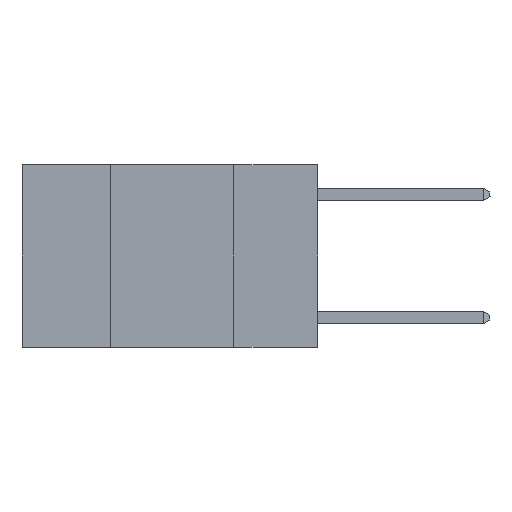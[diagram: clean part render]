
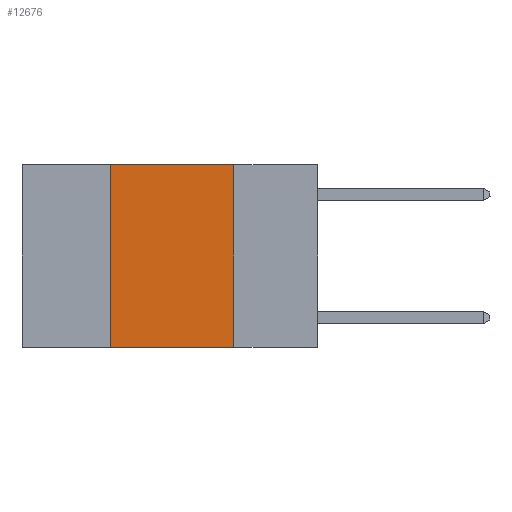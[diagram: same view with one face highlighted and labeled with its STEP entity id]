
A CAD part, left-side view. The second image highlights one B-rep face of the part: STEP entity #12676.
In plain terms, the highlighted planar face has unit normal (-1, 0, 0).
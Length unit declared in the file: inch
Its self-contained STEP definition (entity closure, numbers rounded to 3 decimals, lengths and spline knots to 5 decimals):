
#191 = DIRECTION ( 'NONE',  ( 0., -1., 0. ) ) ;
#1680 = DIRECTION ( 'NONE',  ( 0., 0., 1. ) ) ;
#1792 = ORIENTED_EDGE ( 'NONE', *, *, #13717, .F. ) ;
#2006 = CARTESIAN_POINT ( 'NONE',  ( 0., 0.17, 0. ) ) ;
#2585 = LINE ( 'NONE', #7624, #8014 ) ;
#2943 = FACE_OUTER_BOUND ( 'NONE', #9807, .T. ) ;
#3762 = VECTOR ( 'NONE', #191, 39.37008 ) ;
#3884 = DIRECTION ( 'NONE',  ( 1., 0., 0. ) ) ;
#4231 = AXIS2_PLACEMENT_3D ( 'NONE', #13083, #3884, #7622 ) ;
#4232 = DIRECTION ( 'NONE',  ( 0., 0., -1. ) ) ;
#5155 = CARTESIAN_POINT ( 'NONE',  ( 0., 0.42, 0. ) ) ;
#5337 = VERTEX_POINT ( 'NONE', #11431 ) ;
#5455 = PLANE ( 'NONE',  #4231 ) ;
#6444 = EDGE_CURVE ( 'NONE', #10945, #5337, #6558, .T. ) ;
#6558 = LINE ( 'NONE', #2006, #12008 ) ;
#6949 = ORIENTED_EDGE ( 'NONE', *, *, #6444, .F. ) ;
#7285 = ORIENTED_EDGE ( 'NONE', *, *, #8352, .T. ) ;
#7622 = DIRECTION ( 'NONE',  ( 0., 0., -1. ) ) ;
#7624 = CARTESIAN_POINT ( 'NONE',  ( 0., 0.6, -0.37 ) ) ;
#7993 = CARTESIAN_POINT ( 'NONE',  ( 0., 0.42, -0.37 ) ) ;
#8014 = VECTOR ( 'NONE', #8740, 39.37008 ) ;
#8352 = EDGE_CURVE ( 'NONE', #13600, #5337, #2585, .T. ) ;
#8740 = DIRECTION ( 'NONE',  ( 0., -1., 0. ) ) ;
#9133 = VERTEX_POINT ( 'NONE', #5155 ) ;
#9337 = CARTESIAN_POINT ( 'NONE',  ( 0., 0.42, 0. ) ) ;
#9434 = EDGE_CURVE ( 'NONE', #9133, #10945, #9532, .T. ) ;
#9532 = LINE ( 'NONE', #13301, #3762 ) ;
#9807 = EDGE_LOOP ( 'NONE', ( #6949, #10526, #1792, #7285 ) ) ;
#9883 = LINE ( 'NONE', #9337, #12441 ) ;
#10526 = ORIENTED_EDGE ( 'NONE', *, *, #9434, .F. ) ;
#10945 = VERTEX_POINT ( 'NONE', #11532 ) ;
#11431 = CARTESIAN_POINT ( 'NONE',  ( 0., 0.17, -0.37 ) ) ;
#11532 = CARTESIAN_POINT ( 'NONE',  ( 0., 0.17, 0. ) ) ;
#12008 = VECTOR ( 'NONE', #4232, 39.37008 ) ;
#12441 = VECTOR ( 'NONE', #1680, 39.37008 ) ;
#12676 = ADVANCED_FACE ( 'NONE', ( #2943 ), #5455, .F. ) ;
#13083 = CARTESIAN_POINT ( 'NONE',  ( 0., 0.6, 0. ) ) ;
#13301 = CARTESIAN_POINT ( 'NONE',  ( 0., 0.6, 0. ) ) ;
#13600 = VERTEX_POINT ( 'NONE', #7993 ) ;
#13717 = EDGE_CURVE ( 'NONE', #13600, #9133, #9883, .T. ) ;
